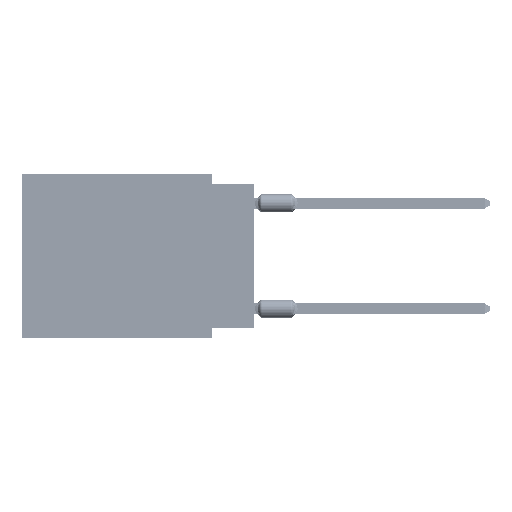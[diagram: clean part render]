
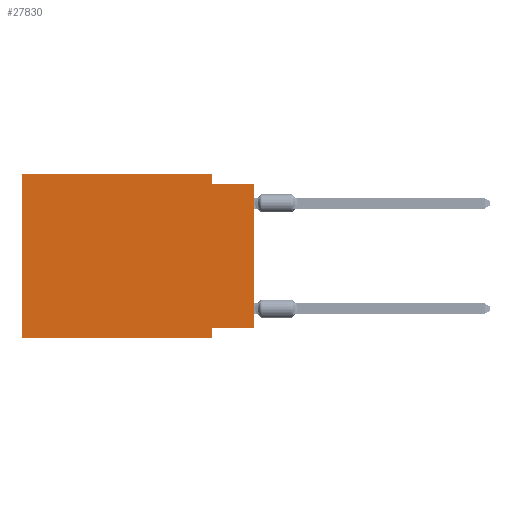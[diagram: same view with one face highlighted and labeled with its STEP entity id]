
A CAD part, left-side view. The second image highlights one B-rep face of the part: STEP entity #27830.
In plain terms, the highlighted planar face has unit normal (-1, 0, 0).
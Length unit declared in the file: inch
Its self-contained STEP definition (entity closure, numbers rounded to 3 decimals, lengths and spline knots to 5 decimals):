
#3053 = CARTESIAN_POINT ( 'NONE',  ( 0., 0., -0.025 ) ) ;
#6511 = CARTESIAN_POINT ( 'NONE',  ( 0., 0.1, 0. ) ) ;
#7465 = CARTESIAN_POINT ( 'NONE',  ( 0., 0., -0.365 ) ) ;
#9307 = CARTESIAN_POINT ( 'NONE',  ( 0., 0.55, 0. ) ) ;
#9640 = LINE ( 'NONE', #64654, #46862 ) ;
#11247 = PLANE ( 'NONE',  #17220 ) ;
#13196 = CARTESIAN_POINT ( 'NONE',  ( 0., 0.1, -0.39 ) ) ;
#15356 = CARTESIAN_POINT ( 'NONE',  ( 0., 0., -0.365 ) ) ;
#15679 = CARTESIAN_POINT ( 'NONE',  ( 0., 0.1, -0.39 ) ) ;
#16486 = LINE ( 'NONE', #15679, #30968 ) ;
#17078 = LINE ( 'NONE', #3053, #80476 ) ;
#17192 = VERTEX_POINT ( 'NONE', #6511 ) ;
#17211 = CARTESIAN_POINT ( 'NONE',  ( 0., 0.55, 0. ) ) ;
#17220 = AXIS2_PLACEMENT_3D ( 'NONE', #62094, #73650, #67874 ) ;
#17366 = ORIENTED_EDGE ( 'NONE', *, *, #61832, .F. ) ;
#17831 = VECTOR ( 'NONE', #22979, 39.37008 ) ;
#18616 = EDGE_CURVE ( 'NONE', #76646, #17192, #29586, .T. ) ;
#18671 = VERTEX_POINT ( 'NONE', #42021 ) ;
#18793 = EDGE_CURVE ( 'NONE', #21469, #56954, #81224, .T. ) ;
#18959 = CARTESIAN_POINT ( 'NONE',  ( 0., 0.55, 0. ) ) ;
#19946 = CARTESIAN_POINT ( 'NONE',  ( 0., 0.1, -0.365 ) ) ;
#21469 = VERTEX_POINT ( 'NONE', #47178 ) ;
#22979 = DIRECTION ( 'NONE',  ( 0., -1., 0. ) ) ;
#23202 = ORIENTED_EDGE ( 'NONE', *, *, #78745, .T. ) ;
#24201 = CARTESIAN_POINT ( 'NONE',  ( 0., 0.55, -0.39 ) ) ;
#27830 = ADVANCED_FACE ( 'NONE', ( #61682 ), #11247, .F. ) ;
#29043 = ORIENTED_EDGE ( 'NONE', *, *, #70987, .F. ) ;
#29586 = LINE ( 'NONE', #17211, #17831 ) ;
#30968 = VECTOR ( 'NONE', #35466, 39.37008 ) ;
#31388 = VECTOR ( 'NONE', #41949, 39.37008 ) ;
#33628 = DIRECTION ( 'NONE',  ( 0., 0., 1. ) ) ;
#34255 = LINE ( 'NONE', #72679, #75108 ) ;
#35466 = DIRECTION ( 'NONE',  ( 0., 0., -1. ) ) ;
#36113 = CARTESIAN_POINT ( 'NONE',  ( 0., 0., -0.025 ) ) ;
#37261 = EDGE_CURVE ( 'NONE', #81125, #50772, #38873, .T. ) ;
#37392 = DIRECTION ( 'NONE',  ( 0., -1., 0. ) ) ;
#38873 = LINE ( 'NONE', #7465, #57157 ) ;
#40724 = LINE ( 'NONE', #9307, #31388 ) ;
#40862 = ORIENTED_EDGE ( 'NONE', *, *, #18616, .F. ) ;
#41949 = DIRECTION ( 'NONE',  ( 0., 0., 1. ) ) ;
#42021 = CARTESIAN_POINT ( 'NONE',  ( 0., 0.1, -0.025 ) ) ;
#46862 = VECTOR ( 'NONE', #33628, 39.37008 ) ;
#46944 = VERTEX_POINT ( 'NONE', #36113 ) ;
#47178 = CARTESIAN_POINT ( 'NONE',  ( 0., 0.55, -0.39 ) ) ;
#49552 = VECTOR ( 'NONE', #37392, 39.37008 ) ;
#50251 = ORIENTED_EDGE ( 'NONE', *, *, #51790, .F. ) ;
#50772 = VERTEX_POINT ( 'NONE', #19946 ) ;
#51790 = EDGE_CURVE ( 'NONE', #21469, #76646, #40724, .T. ) ;
#53164 = EDGE_LOOP ( 'NONE', ( #23202, #59965, #29043, #40862, #50251, #74319, #17366, #74418 ) ) ;
#53483 = DIRECTION ( 'NONE',  ( 0., -1., 0. ) ) ;
#56954 = VERTEX_POINT ( 'NONE', #13196 ) ;
#57157 = VECTOR ( 'NONE', #64095, 39.37008 ) ;
#59965 = ORIENTED_EDGE ( 'NONE', *, *, #74046, .F. ) ;
#61682 = FACE_OUTER_BOUND ( 'NONE', #53164, .T. ) ;
#61832 = EDGE_CURVE ( 'NONE', #50772, #56954, #16486, .T. ) ;
#62094 = CARTESIAN_POINT ( 'NONE',  ( 0., 0.55, 0. ) ) ;
#64095 = DIRECTION ( 'NONE',  ( 0., 1., 0. ) ) ;
#64654 = CARTESIAN_POINT ( 'NONE',  ( 0., 0., 0. ) ) ;
#67874 = DIRECTION ( 'NONE',  ( 0., 0., -1. ) ) ;
#70987 = EDGE_CURVE ( 'NONE', #17192, #18671, #34255, .T. ) ;
#72679 = CARTESIAN_POINT ( 'NONE',  ( 0., 0.1, 0. ) ) ;
#73077 = DIRECTION ( 'NONE',  ( 0., 0., -1. ) ) ;
#73650 = DIRECTION ( 'NONE',  ( 1., 0., 0. ) ) ;
#74046 = EDGE_CURVE ( 'NONE', #18671, #46944, #17078, .T. ) ;
#74319 = ORIENTED_EDGE ( 'NONE', *, *, #18793, .T. ) ;
#74418 = ORIENTED_EDGE ( 'NONE', *, *, #37261, .F. ) ;
#75108 = VECTOR ( 'NONE', #73077, 39.37008 ) ;
#76646 = VERTEX_POINT ( 'NONE', #18959 ) ;
#78745 = EDGE_CURVE ( 'NONE', #81125, #46944, #9640, .T. ) ;
#80476 = VECTOR ( 'NONE', #53483, 39.37008 ) ;
#81125 = VERTEX_POINT ( 'NONE', #15356 ) ;
#81224 = LINE ( 'NONE', #24201, #49552 ) ;
